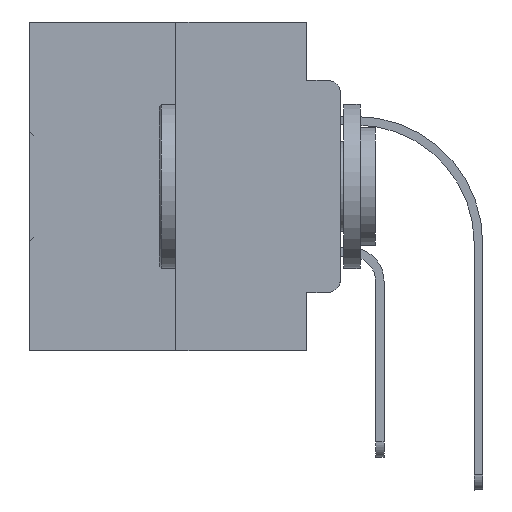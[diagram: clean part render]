
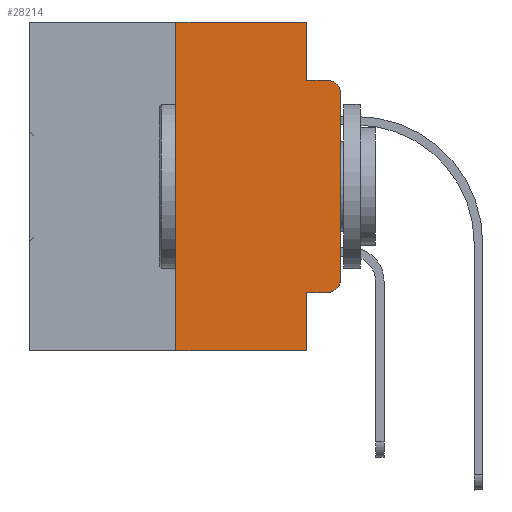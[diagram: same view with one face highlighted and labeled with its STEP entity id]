
A CAD part, left-side view. The second image highlights one B-rep face of the part: STEP entity #28214.
In plain terms, the highlighted planar face has unit normal (-1, 0, 0).
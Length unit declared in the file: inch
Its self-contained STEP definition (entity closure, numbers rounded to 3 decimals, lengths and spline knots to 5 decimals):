
#102 = LINE ( 'NONE', #5918, #35179 ) ;
#549 = LINE ( 'NONE', #24997, #5094 ) ;
#561 = AXIS2_PLACEMENT_3D ( 'NONE', #19217, #33788, #11168 ) ;
#581 = VERTEX_POINT ( 'NONE', #4696 ) ;
#923 = EDGE_LOOP ( 'NONE', ( #22116, #15216, #35591, #33656, #3902, #21408, #26866, #26245, #5276, #29996 ) ) ;
#1990 = LINE ( 'NONE', #35378, #34848 ) ;
#2006 = AXIS2_PLACEMENT_3D ( 'NONE', #34660, #9650, #15501 ) ;
#2559 = CARTESIAN_POINT ( 'NONE',  ( 0., 0.051, -0.0885 ) ) ;
#2761 = LINE ( 'NONE', #30856, #33643 ) ;
#3655 = EDGE_CURVE ( 'NONE', #30008, #29203, #19318, .T. ) ;
#3802 = CARTESIAN_POINT ( 'NONE',  ( 0., 0.051, -0.5 ) ) ;
#3891 = VERTEX_POINT ( 'NONE', #4852 ) ;
#3902 = ORIENTED_EDGE ( 'NONE', *, *, #9982, .F. ) ;
#3917 = AXIS2_PLACEMENT_3D ( 'NONE', #10746, #35578, #8006 ) ;
#4696 = CARTESIAN_POINT ( 'NONE',  ( 0., 0., -0.3915 ) ) ;
#4852 = CARTESIAN_POINT ( 'NONE',  ( 0., 0., -0.1085 ) ) ;
#4871 = CIRCLE ( 'NONE', #2006, 0.02 ) ;
#5094 = VECTOR ( 'NONE', #5648, 39.37008 ) ;
#5259 = DIRECTION ( 'NONE',  ( 0., 0., 1. ) ) ;
#5275 = CARTESIAN_POINT ( 'NONE',  ( 0., 0.051, -0.4115 ) ) ;
#5276 = ORIENTED_EDGE ( 'NONE', *, *, #21207, .T. ) ;
#5568 = DIRECTION ( 'NONE',  ( 0., -1., 0. ) ) ;
#5648 = DIRECTION ( 'NONE',  ( 0., 0., -1. ) ) ;
#5796 = CARTESIAN_POINT ( 'NONE',  ( 0., 0.25, 0. ) ) ;
#5918 = CARTESIAN_POINT ( 'NONE',  ( 0., 0.051, -0.4115 ) ) ;
#6317 = CARTESIAN_POINT ( 'NONE',  ( 0., 0.051, 0. ) ) ;
#7303 = CARTESIAN_POINT ( 'NONE',  ( 0., 0.473, 0. ) ) ;
#8006 = DIRECTION ( 'NONE',  ( 0., 0., -1. ) ) ;
#9650 = DIRECTION ( 'NONE',  ( -1., 0., 0. ) ) ;
#9982 = EDGE_CURVE ( 'NONE', #29203, #14533, #12595, .T. ) ;
#10375 = DIRECTION ( 'NONE',  ( 0., -1., 0. ) ) ;
#10746 = CARTESIAN_POINT ( 'NONE',  ( 0., 0.473, 0. ) ) ;
#10788 = LINE ( 'NONE', #16446, #20190 ) ;
#11168 = DIRECTION ( 'NONE',  ( 0., 0., -1. ) ) ;
#11570 = VERTEX_POINT ( 'NONE', #20049 ) ;
#11848 = LINE ( 'NONE', #12390, #19089 ) ;
#11969 = EDGE_CURVE ( 'NONE', #3891, #17209, #31448, .T. ) ;
#12112 = VECTOR ( 'NONE', #16071, 39.37008 ) ;
#12390 = CARTESIAN_POINT ( 'NONE',  ( 0., 0.051, -0.0885 ) ) ;
#12410 = VERTEX_POINT ( 'NONE', #2559 ) ;
#12595 = LINE ( 'NONE', #7303, #12112 ) ;
#12669 = VERTEX_POINT ( 'NONE', #3802 ) ;
#14533 = VERTEX_POINT ( 'NONE', #6317 ) ;
#14910 = CARTESIAN_POINT ( 'NONE',  ( 0., 0.02, -0.0885 ) ) ;
#15216 = ORIENTED_EDGE ( 'NONE', *, *, #11969, .T. ) ;
#15501 = DIRECTION ( 'NONE',  ( 0., 0., -1. ) ) ;
#16071 = DIRECTION ( 'NONE',  ( 0., -1., 0. ) ) ;
#16446 = CARTESIAN_POINT ( 'NONE',  ( 0., 0.051, 0. ) ) ;
#17209 = VERTEX_POINT ( 'NONE', #14910 ) ;
#17589 = CARTESIAN_POINT ( 'NONE',  ( 0., 0.25, 0. ) ) ;
#19089 = VECTOR ( 'NONE', #31387, 39.37008 ) ;
#19217 = CARTESIAN_POINT ( 'NONE',  ( 0., 0.02, -0.1085 ) ) ;
#19318 = LINE ( 'NONE', #5796, #21938 ) ;
#19535 = DIRECTION ( 'NONE',  ( 0., 0., 1. ) ) ;
#20049 = CARTESIAN_POINT ( 'NONE',  ( 0., 0.02, -0.4115 ) ) ;
#20190 = VECTOR ( 'NONE', #32703, 39.37008 ) ;
#21207 = EDGE_CURVE ( 'NONE', #35575, #11570, #102, .T. ) ;
#21408 = ORIENTED_EDGE ( 'NONE', *, *, #3655, .F. ) ;
#21827 = EDGE_CURVE ( 'NONE', #11570, #581, #4871, .T. ) ;
#21938 = VECTOR ( 'NONE', #5259, 39.37008 ) ;
#22116 = ORIENTED_EDGE ( 'NONE', *, *, #27968, .T. ) ;
#24997 = CARTESIAN_POINT ( 'NONE',  ( 0., 0.051, 0. ) ) ;
#26245 = ORIENTED_EDGE ( 'NONE', *, *, #26622, .F. ) ;
#26622 = EDGE_CURVE ( 'NONE', #35575, #12669, #549, .T. ) ;
#26866 = ORIENTED_EDGE ( 'NONE', *, *, #26981, .T. ) ;
#26981 = EDGE_CURVE ( 'NONE', #30008, #12669, #1990, .T. ) ;
#27758 = EDGE_CURVE ( 'NONE', #14533, #12410, #10788, .T. ) ;
#27968 = EDGE_CURVE ( 'NONE', #581, #3891, #2761, .T. ) ;
#28064 = EDGE_CURVE ( 'NONE', #12410, #17209, #11848, .T. ) ;
#28214 = ADVANCED_FACE ( 'NONE', ( #32833 ), #32471, .F. ) ;
#28215 = CARTESIAN_POINT ( 'NONE',  ( 0., 0.25, -0.5 ) ) ;
#29203 = VERTEX_POINT ( 'NONE', #17589 ) ;
#29996 = ORIENTED_EDGE ( 'NONE', *, *, #21827, .T. ) ;
#30008 = VERTEX_POINT ( 'NONE', #28215 ) ;
#30856 = CARTESIAN_POINT ( 'NONE',  ( 0., 0., 0. ) ) ;
#31387 = DIRECTION ( 'NONE',  ( 0., -1., 0. ) ) ;
#31448 = CIRCLE ( 'NONE', #561, 0.02 ) ;
#32471 = PLANE ( 'NONE',  #3917 ) ;
#32703 = DIRECTION ( 'NONE',  ( 0., 0., -1. ) ) ;
#32833 = FACE_OUTER_BOUND ( 'NONE', #923, .T. ) ;
#33643 = VECTOR ( 'NONE', #19535, 39.37008 ) ;
#33656 = ORIENTED_EDGE ( 'NONE', *, *, #27758, .F. ) ;
#33788 = DIRECTION ( 'NONE',  ( -1., 0., 0. ) ) ;
#34660 = CARTESIAN_POINT ( 'NONE',  ( 0., 0.02, -0.3915 ) ) ;
#34848 = VECTOR ( 'NONE', #10375, 39.37008 ) ;
#35179 = VECTOR ( 'NONE', #5568, 39.37008 ) ;
#35378 = CARTESIAN_POINT ( 'NONE',  ( 0., 0.473, -0.5 ) ) ;
#35575 = VERTEX_POINT ( 'NONE', #5275 ) ;
#35578 = DIRECTION ( 'NONE',  ( 1., 0., 0. ) ) ;
#35591 = ORIENTED_EDGE ( 'NONE', *, *, #28064, .F. ) ;
